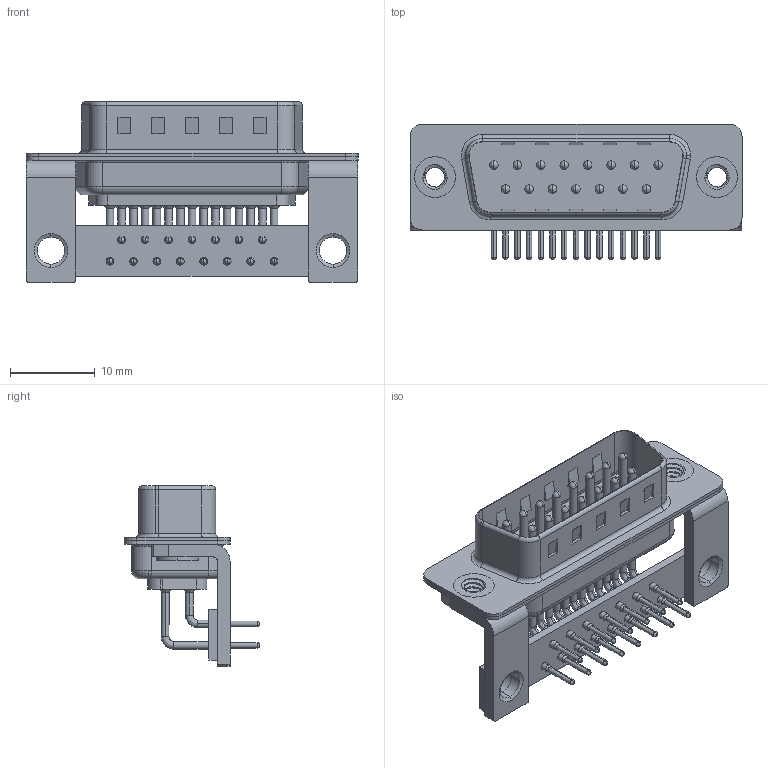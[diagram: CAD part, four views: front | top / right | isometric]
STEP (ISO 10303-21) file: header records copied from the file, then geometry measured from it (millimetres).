
FILE_DESCRIPTION (( 'STEP AP203' ), '1' );
FILE_NAME ('629-M15-340-GN4.STEP', '2018-09-25T17:43:26', ( '' ), ( '' ), 'SwSTEP 2.0', 'SolidWorks 2016', '' );
FILE_SCHEMA (( 'CONFIG_CONTROL_DESIGN' ));
Length unit declared in the file: millimetre
Products named in the file (9): 629M Shell Rear_15 Contacts; 629M Contact Row 1; 629M Contact Row 2; 629M 4-40 Threaded Rivet_Stabilizer; 629M Housing_15 Contacts; 629M Stabilizer Bracket; 629M Shell Front_15 Contacts; 629M Stabilizer Board_15 Contacts; 629-M15-340-GN4
Assembly tree (23 placements, depth 2):
  629-M15-340-GN4
    629M Housing_15 Contacts
    629M Shell Front_15 Contacts
    629M Shell Rear_15 Contacts
    629M Contact Row 1  x8
    629M Contact Row 2  x7
    629M 4-40 Threaded Rivet_Stabilizer  x2
    629M Stabilizer Bracket  x2
    629M Stabilizer Board_15 Contacts
Bounding box: 39.2 x 16 x 21.3 mm (x, y, z)
Volume: 2435 mm3; surface area: 6519.3 mm2
Topology: 23 solids, 23 shells, 2070 faces, 5745 edges, 3732 vertices
Faces by surface type: plane 1125, cylinder 725, bspline 96, cone 68, torus 56
Entity records: 24377 total; most frequent: CARTESIAN_POINT 5345, DIRECTION 3859, ORIENTED_EDGE 3584, EDGE_CURVE 1792, AXIS2_PLACEMENT_3D 1408, VERTEX_POINT 1160, VECTOR 1043, LINE 1043
